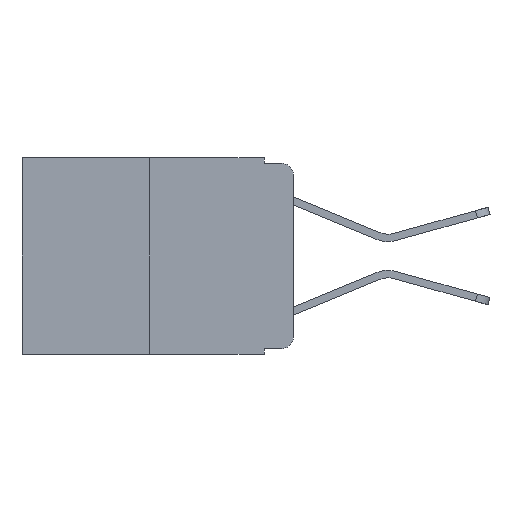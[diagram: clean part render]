
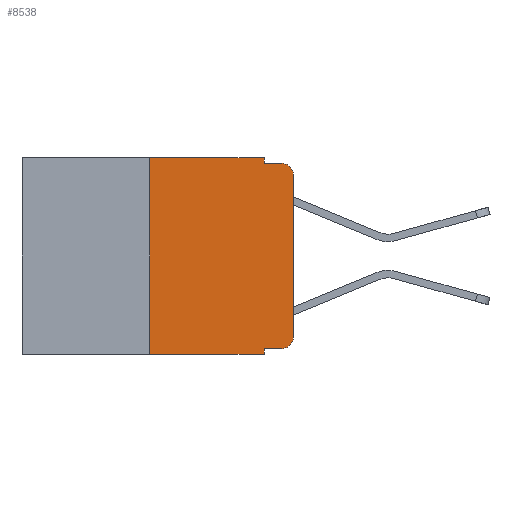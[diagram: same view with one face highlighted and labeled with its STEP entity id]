
A CAD part, left-side view. The second image highlights one B-rep face of the part: STEP entity #8538.
In plain terms, the highlighted planar face has unit normal (-1, 0, 0).
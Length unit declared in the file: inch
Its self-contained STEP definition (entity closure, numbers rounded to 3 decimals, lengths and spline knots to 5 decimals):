
#58 = DIRECTION ( 'NONE',  ( 0., -1., 0. ) ) ;
#268 = AXIS2_PLACEMENT_3D ( 'NONE', #17595, #9274, #339 ) ;
#275 = PLANE ( 'NONE',  #11502 ) ;
#338 = CARTESIAN_POINT ( 'NONE',  ( 0., 0.473, 0. ) ) ;
#339 = DIRECTION ( 'NONE',  ( 0., 0., -1. ) ) ;
#365 = VECTOR ( 'NONE', #2261, 39.37008 ) ;
#382 = CARTESIAN_POINT ( 'NONE',  ( 0., 0.25, 0. ) ) ;
#506 = VERTEX_POINT ( 'NONE', #11730 ) ;
#570 = DIRECTION ( 'NONE',  ( 0., 0., -1. ) ) ;
#592 = DIRECTION ( 'NONE',  ( 1., 0., 0. ) ) ;
#661 = VERTEX_POINT ( 'NONE', #4782 ) ;
#906 = EDGE_CURVE ( 'NONE', #13333, #3483, #14711, .T. ) ;
#933 = DIRECTION ( 'NONE',  ( 0., 0., -1. ) ) ;
#1184 = CARTESIAN_POINT ( 'NONE',  ( 0., 0.02, -0.01 ) ) ;
#1240 = ORIENTED_EDGE ( 'NONE', *, *, #2957, .F. ) ;
#1405 = CARTESIAN_POINT ( 'NONE',  ( 0., 0.051, -0.01 ) ) ;
#1736 = VERTEX_POINT ( 'NONE', #11729 ) ;
#1786 = ORIENTED_EDGE ( 'NONE', *, *, #17642, .T. ) ;
#1980 = DIRECTION ( 'NONE',  ( 0., -1., 0. ) ) ;
#2261 = DIRECTION ( 'NONE',  ( 0., 0., 1. ) ) ;
#2957 = EDGE_CURVE ( 'NONE', #13333, #1736, #3957, .T. ) ;
#2990 = EDGE_CURVE ( 'NONE', #16282, #1736, #10725, .T. ) ;
#3179 = CARTESIAN_POINT ( 'NONE',  ( 0., 0.473, 0. ) ) ;
#3319 = CARTESIAN_POINT ( 'NONE',  ( 0., 0.051, -0.333 ) ) ;
#3338 = VERTEX_POINT ( 'NONE', #3684 ) ;
#3372 = ORIENTED_EDGE ( 'NONE', *, *, #15416, .T. ) ;
#3483 = VERTEX_POINT ( 'NONE', #17055 ) ;
#3492 = VECTOR ( 'NONE', #11170, 39.37008 ) ;
#3684 = CARTESIAN_POINT ( 'NONE',  ( 0., 0., -0.313 ) ) ;
#3845 = DIRECTION ( 'NONE',  ( 0., 0., -1. ) ) ;
#3853 = ORIENTED_EDGE ( 'NONE', *, *, #2990, .T. ) ;
#3957 = LINE ( 'NONE', #13669, #11166 ) ;
#4275 = VECTOR ( 'NONE', #18315, 39.37008 ) ;
#4782 = CARTESIAN_POINT ( 'NONE',  ( 0., 0.051, 0. ) ) ;
#4807 = ORIENTED_EDGE ( 'NONE', *, *, #14481, .T. ) ;
#5058 = LINE ( 'NONE', #9617, #12619 ) ;
#6135 = CARTESIAN_POINT ( 'NONE',  ( 0., 0.051, -0.01 ) ) ;
#6518 = FACE_OUTER_BOUND ( 'NONE', #18375, .T. ) ;
#6668 = ORIENTED_EDGE ( 'NONE', *, *, #12623, .F. ) ;
#7775 = ORIENTED_EDGE ( 'NONE', *, *, #906, .T. ) ;
#7949 = EDGE_CURVE ( 'NONE', #16282, #12729, #8340, .T. ) ;
#8003 = LINE ( 'NONE', #6135, #11271 ) ;
#8238 = AXIS2_PLACEMENT_3D ( 'NONE', #18119, #9784, #933 ) ;
#8340 = LINE ( 'NONE', #382, #365 ) ;
#8538 = ADVANCED_FACE ( 'NONE', ( #6518 ), #275, .F. ) ;
#8669 = EDGE_CURVE ( 'NONE', #12729, #661, #12249, .T. ) ;
#9274 = DIRECTION ( 'NONE',  ( -1., 0., 0. ) ) ;
#9617 = CARTESIAN_POINT ( 'NONE',  ( 0., 0.051, 0. ) ) ;
#9761 = ORIENTED_EDGE ( 'NONE', *, *, #8669, .F. ) ;
#9784 = DIRECTION ( 'NONE',  ( -1., 0., 0. ) ) ;
#10265 = CARTESIAN_POINT ( 'NONE',  ( 0., 0.051, -0.333 ) ) ;
#10725 = LINE ( 'NONE', #16259, #14434 ) ;
#10922 = VECTOR ( 'NONE', #1980, 39.37008 ) ;
#11166 = VECTOR ( 'NONE', #13624, 39.37008 ) ;
#11170 = DIRECTION ( 'NONE',  ( 0., 0., 1. ) ) ;
#11189 = LINE ( 'NONE', #18107, #3492 ) ;
#11271 = VECTOR ( 'NONE', #58, 39.37008 ) ;
#11502 = AXIS2_PLACEMENT_3D ( 'NONE', #3179, #592, #570 ) ;
#11684 = EDGE_CURVE ( 'NONE', #661, #16866, #5058, .T. ) ;
#11729 = CARTESIAN_POINT ( 'NONE',  ( 0., 0.051, -0.343 ) ) ;
#11730 = CARTESIAN_POINT ( 'NONE',  ( 0., 0., -0.03 ) ) ;
#12249 = LINE ( 'NONE', #338, #10922 ) ;
#12342 = CIRCLE ( 'NONE', #8238, 0.02 ) ;
#12537 = CIRCLE ( 'NONE', #268, 0.02 ) ;
#12619 = VECTOR ( 'NONE', #3845, 39.37008 ) ;
#12623 = EDGE_CURVE ( 'NONE', #16866, #18399, #8003, .T. ) ;
#12729 = VERTEX_POINT ( 'NONE', #13332 ) ;
#13032 = ORIENTED_EDGE ( 'NONE', *, *, #11684, .F. ) ;
#13332 = CARTESIAN_POINT ( 'NONE',  ( 0., 0.25, 0. ) ) ;
#13333 = VERTEX_POINT ( 'NONE', #3319 ) ;
#13624 = DIRECTION ( 'NONE',  ( 0., 0., -1. ) ) ;
#13669 = CARTESIAN_POINT ( 'NONE',  ( 0., 0.051, 0. ) ) ;
#14434 = VECTOR ( 'NONE', #18192, 39.37008 ) ;
#14481 = EDGE_CURVE ( 'NONE', #506, #18399, #12537, .T. ) ;
#14711 = LINE ( 'NONE', #10265, #4275 ) ;
#15416 = EDGE_CURVE ( 'NONE', #3338, #506, #11189, .T. ) ;
#15826 = CARTESIAN_POINT ( 'NONE',  ( 0., 0.25, -0.343 ) ) ;
#16259 = CARTESIAN_POINT ( 'NONE',  ( 0., 0.473, -0.343 ) ) ;
#16282 = VERTEX_POINT ( 'NONE', #15826 ) ;
#16866 = VERTEX_POINT ( 'NONE', #1405 ) ;
#17055 = CARTESIAN_POINT ( 'NONE',  ( 0., 0.02, -0.333 ) ) ;
#17595 = CARTESIAN_POINT ( 'NONE',  ( 0., 0.02, -0.03 ) ) ;
#17642 = EDGE_CURVE ( 'NONE', #3483, #3338, #12342, .T. ) ;
#18051 = ORIENTED_EDGE ( 'NONE', *, *, #7949, .F. ) ;
#18107 = CARTESIAN_POINT ( 'NONE',  ( 0., 0., 0. ) ) ;
#18119 = CARTESIAN_POINT ( 'NONE',  ( 0., 0.02, -0.313 ) ) ;
#18192 = DIRECTION ( 'NONE',  ( 0., -1., 0. ) ) ;
#18315 = DIRECTION ( 'NONE',  ( 0., -1., 0. ) ) ;
#18375 = EDGE_LOOP ( 'NONE', ( #3372, #4807, #6668, #13032, #9761, #18051, #3853, #1240, #7775, #1786 ) ) ;
#18399 = VERTEX_POINT ( 'NONE', #1184 ) ;
